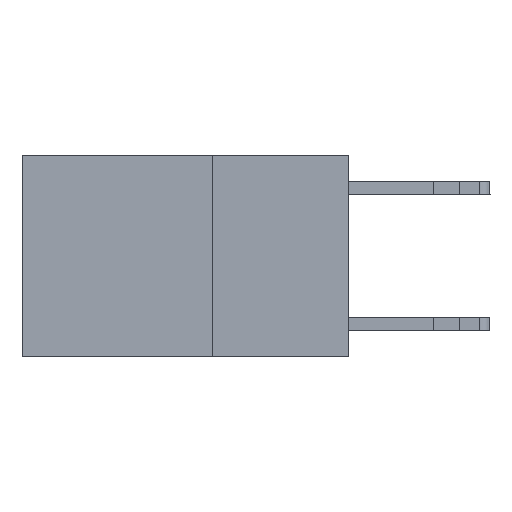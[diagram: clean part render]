
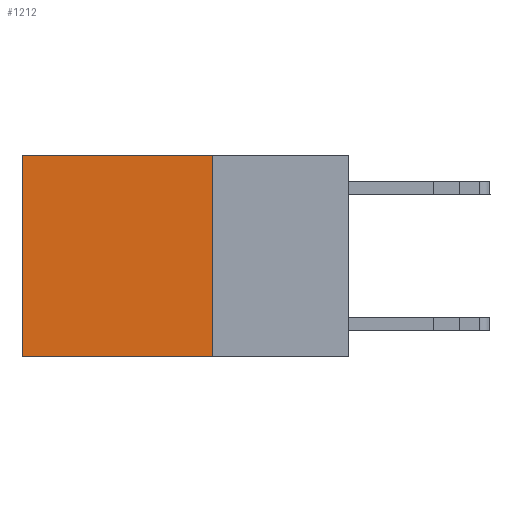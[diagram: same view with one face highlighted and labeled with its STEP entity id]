
A CAD part, left-side view. The second image highlights one B-rep face of the part: STEP entity #1212.
In plain terms, the highlighted planar face has unit normal (-1, 0, 0).
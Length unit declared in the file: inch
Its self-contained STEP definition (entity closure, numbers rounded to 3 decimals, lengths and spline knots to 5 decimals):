
#291 = VECTOR ( 'NONE', #8582, 39.37008 ) ;
#469 = CARTESIAN_POINT ( 'NONE',  ( 0.2625, 0.25, 0. ) ) ;
#1212 = ADVANCED_FACE ( 'NONE', ( #10147 ), #15947, .F. ) ;
#1607 = DIRECTION ( 'NONE',  ( 0., 0., -1. ) ) ;
#2795 = EDGE_LOOP ( 'NONE', ( #14264, #3096, #5744, #5867 ) ) ;
#2804 = LINE ( 'NONE', #17379, #18213 ) ;
#2960 = EDGE_CURVE ( 'NONE', #18534, #7318, #8940, .T. ) ;
#3057 = DIRECTION ( 'NONE',  ( 1., 0., 0. ) ) ;
#3096 = ORIENTED_EDGE ( 'NONE', *, *, #2960, .F. ) ;
#3389 = VERTEX_POINT ( 'NONE', #11652 ) ;
#5744 = ORIENTED_EDGE ( 'NONE', *, *, #17029, .F. ) ;
#5867 = ORIENTED_EDGE ( 'NONE', *, *, #12145, .T. ) ;
#7318 = VERTEX_POINT ( 'NONE', #10453 ) ;
#7457 = EDGE_CURVE ( 'NONE', #3389, #7318, #17749, .T. ) ;
#8577 = DIRECTION ( 'NONE',  ( 0., 1., 0. ) ) ;
#8582 = DIRECTION ( 'NONE',  ( 0., 1., 0. ) ) ;
#8940 = LINE ( 'NONE', #12050, #291 ) ;
#9231 = DIRECTION ( 'NONE',  ( 0., 0., -1. ) ) ;
#9701 = LINE ( 'NONE', #9890, #16203 ) ;
#9890 = CARTESIAN_POINT ( 'NONE',  ( 0.2625, 0.25, 0. ) ) ;
#10147 = FACE_OUTER_BOUND ( 'NONE', #2795, .T. ) ;
#10324 = CARTESIAN_POINT ( 'NONE',  ( 0.2625, 0.25, 0. ) ) ;
#10453 = CARTESIAN_POINT ( 'NONE',  ( 0.2625, 0.6, -0.37 ) ) ;
#11100 = AXIS2_PLACEMENT_3D ( 'NONE', #10324, #3057, #1607 ) ;
#11652 = CARTESIAN_POINT ( 'NONE',  ( 0.2625, 0.6, 0. ) ) ;
#12050 = CARTESIAN_POINT ( 'NONE',  ( 0.2625, 0.25, -0.37 ) ) ;
#12145 = EDGE_CURVE ( 'NONE', #14334, #3389, #2804, .T. ) ;
#13314 = VECTOR ( 'NONE', #9231, 39.37008 ) ;
#13516 = DIRECTION ( 'NONE',  ( 0., 0., -1. ) ) ;
#13583 = CARTESIAN_POINT ( 'NONE',  ( 0.2625, 0.6, 0. ) ) ;
#14264 = ORIENTED_EDGE ( 'NONE', *, *, #7457, .T. ) ;
#14334 = VERTEX_POINT ( 'NONE', #469 ) ;
#15947 = PLANE ( 'NONE',  #11100 ) ;
#16203 = VECTOR ( 'NONE', #13516, 39.37008 ) ;
#17029 = EDGE_CURVE ( 'NONE', #14334, #18534, #9701, .T. ) ;
#17204 = CARTESIAN_POINT ( 'NONE',  ( 0.2625, 0.25, -0.37 ) ) ;
#17379 = CARTESIAN_POINT ( 'NONE',  ( 0.2625, 0.25, 0. ) ) ;
#17749 = LINE ( 'NONE', #13583, #13314 ) ;
#18213 = VECTOR ( 'NONE', #8577, 39.37008 ) ;
#18534 = VERTEX_POINT ( 'NONE', #17204 ) ;
